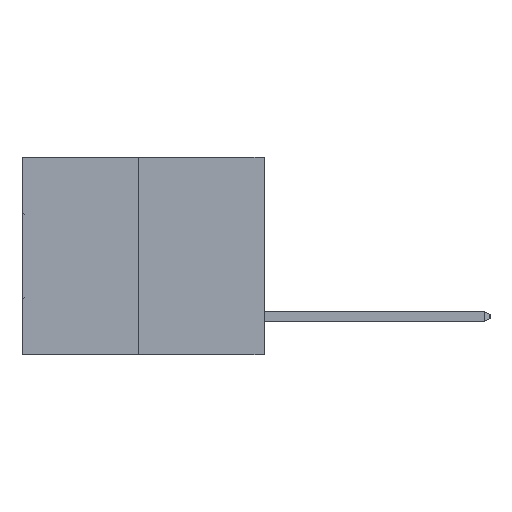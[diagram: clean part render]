
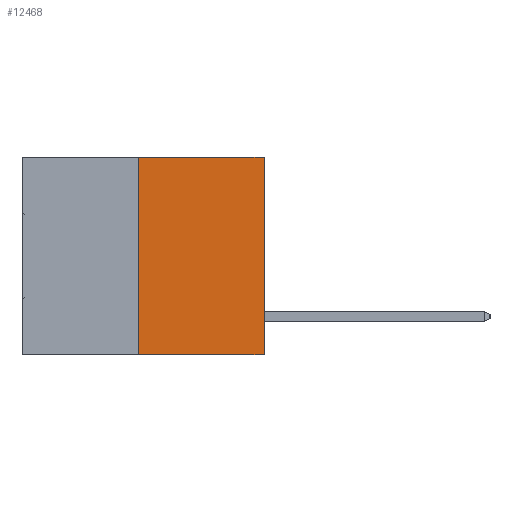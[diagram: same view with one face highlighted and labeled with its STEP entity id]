
A CAD part, left-side view. The second image highlights one B-rep face of the part: STEP entity #12468.
In plain terms, the highlighted planar face has unit normal (-1, 0, 0).
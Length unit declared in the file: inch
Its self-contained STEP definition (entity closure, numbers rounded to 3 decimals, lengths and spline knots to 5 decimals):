
#156 = DIRECTION ( 'NONE',  ( 0., -1., 0. ) ) ;
#639 = VERTEX_POINT ( 'NONE', #32358 ) ;
#1166 = DIRECTION ( 'NONE',  ( 1., 0., 0. ) ) ;
#1313 = CARTESIAN_POINT ( 'NONE',  ( 0., 0.6, -0.49 ) ) ;
#1619 = EDGE_LOOP ( 'NONE', ( #3420, #28057, #9243, #34783 ) ) ;
#3420 = ORIENTED_EDGE ( 'NONE', *, *, #19013, .F. ) ;
#4987 = VECTOR ( 'NONE', #28494, 39.37008 ) ;
#5171 = VERTEX_POINT ( 'NONE', #29488 ) ;
#6696 = CARTESIAN_POINT ( 'NONE',  ( 0., 0.6, 0. ) ) ;
#9243 = ORIENTED_EDGE ( 'NONE', *, *, #16362, .T. ) ;
#12468 = ADVANCED_FACE ( 'NONE', ( #14436 ), #20227, .F. ) ;
#12927 = LINE ( 'NONE', #24755, #31608 ) ;
#13943 = EDGE_CURVE ( 'NONE', #31231, #33174, #21528, .T. ) ;
#14282 = CARTESIAN_POINT ( 'NONE',  ( 0., 0., 0. ) ) ;
#14436 = FACE_OUTER_BOUND ( 'NONE', #1619, .T. ) ;
#15438 = EDGE_CURVE ( 'NONE', #639, #5171, #12927, .T. ) ;
#16362 = EDGE_CURVE ( 'NONE', #33174, #5171, #34071, .T. ) ;
#16756 = VECTOR ( 'NONE', #21443, 39.37008 ) ;
#17075 = VECTOR ( 'NONE', #24610, 39.37008 ) ;
#19013 = EDGE_CURVE ( 'NONE', #31231, #639, #25733, .T. ) ;
#20227 = PLANE ( 'NONE',  #23852 ) ;
#21443 = DIRECTION ( 'NONE',  ( 0., 0., 1. ) ) ;
#21528 = LINE ( 'NONE', #1313, #4987 ) ;
#23852 = AXIS2_PLACEMENT_3D ( 'NONE', #6696, #1166, #25711 ) ;
#24497 = CARTESIAN_POINT ( 'NONE',  ( 0., 0., -0.49 ) ) ;
#24504 = CARTESIAN_POINT ( 'NONE',  ( 0., 0.312, -0.49 ) ) ;
#24610 = DIRECTION ( 'NONE',  ( 0., 0., 1. ) ) ;
#24755 = CARTESIAN_POINT ( 'NONE',  ( 0., 0.6, 0. ) ) ;
#25711 = DIRECTION ( 'NONE',  ( 0., 0., -1. ) ) ;
#25733 = LINE ( 'NONE', #24504, #16756 ) ;
#28057 = ORIENTED_EDGE ( 'NONE', *, *, #13943, .T. ) ;
#28494 = DIRECTION ( 'NONE',  ( 0., -1., 0. ) ) ;
#29488 = CARTESIAN_POINT ( 'NONE',  ( 0., 0., 0. ) ) ;
#31231 = VERTEX_POINT ( 'NONE', #32435 ) ;
#31608 = VECTOR ( 'NONE', #156, 39.37008 ) ;
#32358 = CARTESIAN_POINT ( 'NONE',  ( 0., 0.312, 0. ) ) ;
#32435 = CARTESIAN_POINT ( 'NONE',  ( 0., 0.312, -0.49 ) ) ;
#33174 = VERTEX_POINT ( 'NONE', #24497 ) ;
#34071 = LINE ( 'NONE', #14282, #17075 ) ;
#34783 = ORIENTED_EDGE ( 'NONE', *, *, #15438, .F. ) ;
